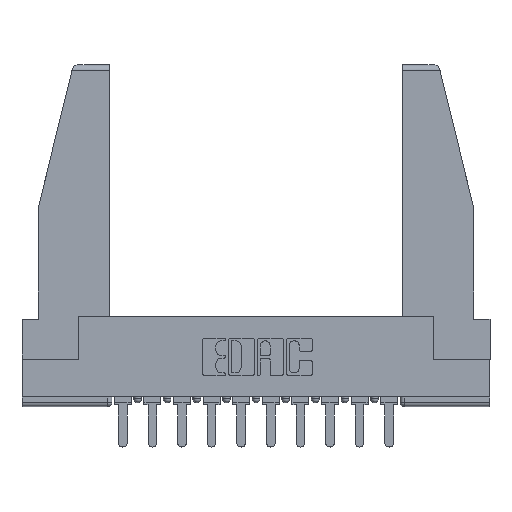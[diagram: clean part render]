
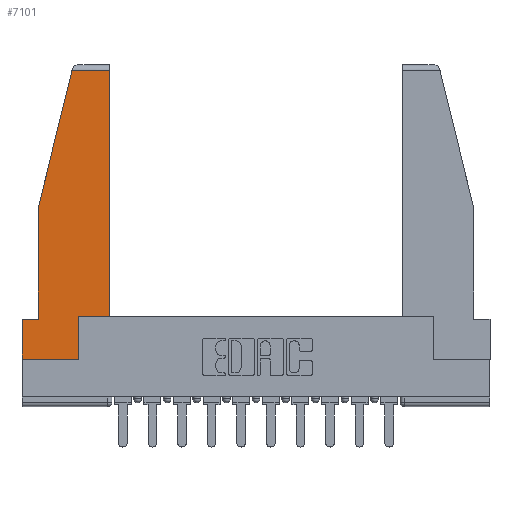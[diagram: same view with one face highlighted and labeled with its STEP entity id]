
A CAD part, top view. The second image highlights one B-rep face of the part: STEP entity #7101.
In plain terms, the highlighted planar face has unit normal (0, 0, 1).
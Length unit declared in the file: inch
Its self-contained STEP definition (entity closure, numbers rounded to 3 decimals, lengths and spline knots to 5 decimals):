
#32 = VERTEX_POINT ( 'NONE', #2172 ) ;
#370 = ORIENTED_EDGE ( 'NONE', *, *, #6871, .T. ) ;
#487 = VERTEX_POINT ( 'NONE', #7999 ) ;
#496 = DIRECTION ( 'NONE',  ( 1., 0., 0. ) ) ;
#651 = CARTESIAN_POINT ( 'NONE',  ( 0.086, 0.21, 0. ) ) ;
#810 = DIRECTION ( 'NONE',  ( 0., -1., 0. ) ) ;
#1042 = ORIENTED_EDGE ( 'NONE', *, *, #3925, .T. ) ;
#1211 = VECTOR ( 'NONE', #810, 39.37008 ) ;
#1615 = LINE ( 'NONE', #4013, #7022 ) ;
#1825 = PLANE ( 'NONE',  #9906 ) ;
#1854 = EDGE_CURVE ( 'NONE', #7035, #11301, #7400, .T. ) ;
#1891 = ORIENTED_EDGE ( 'NONE', *, *, #14746, .T. ) ;
#1901 = DIRECTION ( 'NONE',  ( 0., 0., 1. ) ) ;
#2095 = DIRECTION ( 'NONE',  ( 0., 1., 0. ) ) ;
#2172 = CARTESIAN_POINT ( 'NONE',  ( 0.461, 1.52, 0. ) ) ;
#2199 = VERTEX_POINT ( 'NONE', #10575 ) ;
#2582 = CARTESIAN_POINT ( 'NONE',  ( 0.086, 0.8, 0. ) ) ;
#2620 = DIRECTION ( 'NONE',  ( 0., -1., 0. ) ) ;
#3453 = VERTEX_POINT ( 'NONE', #15131 ) ;
#3714 = ORIENTED_EDGE ( 'NONE', *, *, #15191, .T. ) ;
#3925 = EDGE_CURVE ( 'NONE', #487, #3453, #8111, .T. ) ;
#4013 = CARTESIAN_POINT ( 'NONE',  ( 0.297, 0.223, 0. ) ) ;
#4289 = CARTESIAN_POINT ( 'NONE',  ( 0., 0., 0. ) ) ;
#4654 = VECTOR ( 'NONE', #12395, 39.37008 ) ;
#5049 = EDGE_LOOP ( 'NONE', ( #14803, #5471, #14866, #370, #12545, #3714, #12225, #1042, #1891 ) ) ;
#5052 = DIRECTION ( 'NONE',  ( 0., 1., 0. ) ) ;
#5264 = DIRECTION ( 'NONE',  ( 1., 0., 0. ) ) ;
#5281 = LINE ( 'NONE', #10124, #7884 ) ;
#5455 = DIRECTION ( 'NONE',  ( 1., 0., 0. ) ) ;
#5471 = ORIENTED_EDGE ( 'NONE', *, *, #14448, .T. ) ;
#5668 = CARTESIAN_POINT ( 'NONE',  ( 0.297, 0., 0. ) ) ;
#5722 = LINE ( 'NONE', #6760, #1211 ) ;
#5786 = EDGE_CURVE ( 'NONE', #10288, #487, #11662, .T. ) ;
#5787 = VERTEX_POINT ( 'NONE', #15323 ) ;
#6048 = CARTESIAN_POINT ( 'NONE',  ( 0.086, 0.8, 0. ) ) ;
#6076 = VERTEX_POINT ( 'NONE', #2582 ) ;
#6138 = CARTESIAN_POINT ( 'NONE',  ( 0., 0., 0. ) ) ;
#6269 = VECTOR ( 'NONE', #2095, 39.37008 ) ;
#6735 = LINE ( 'NONE', #14213, #13348 ) ;
#6760 = CARTESIAN_POINT ( 'NONE',  ( 0., 0.21, 0. ) ) ;
#6812 = DIRECTION ( 'NONE',  ( -1., 0., 0. ) ) ;
#6871 = EDGE_CURVE ( 'NONE', #6076, #7035, #11137, .T. ) ;
#6880 = CARTESIAN_POINT ( 'NONE',  ( 0., 0., 0. ) ) ;
#7022 = VECTOR ( 'NONE', #5264, 39.37008 ) ;
#7035 = VERTEX_POINT ( 'NONE', #651 ) ;
#7101 = ADVANCED_FACE ( 'NONE', ( #12695 ), #1825, .T. ) ;
#7369 = EDGE_CURVE ( 'NONE', #5787, #6076, #5281, .T. ) ;
#7400 = LINE ( 'NONE', #7563, #4654 ) ;
#7563 = CARTESIAN_POINT ( 'NONE',  ( 0., 0.21, 0. ) ) ;
#7884 = VECTOR ( 'NONE', #14996, 39.37008 ) ;
#7999 = CARTESIAN_POINT ( 'NONE',  ( 0.297, 0., 0. ) ) ;
#8111 = LINE ( 'NONE', #5668, #6269 ) ;
#9612 = VECTOR ( 'NONE', #5455, 39.37008 ) ;
#9725 = VECTOR ( 'NONE', #5052, 39.37008 ) ;
#9906 = AXIS2_PLACEMENT_3D ( 'NONE', #4289, #1901, #496 ) ;
#10124 = CARTESIAN_POINT ( 'NONE',  ( 0.271, 1.55, 0. ) ) ;
#10288 = VERTEX_POINT ( 'NONE', #6138 ) ;
#10575 = CARTESIAN_POINT ( 'NONE',  ( 0.461, 0.223, 0. ) ) ;
#11137 = LINE ( 'NONE', #6048, #13978 ) ;
#11301 = VERTEX_POINT ( 'NONE', #12149 ) ;
#11662 = LINE ( 'NONE', #6880, #9612 ) ;
#11790 = EDGE_CURVE ( 'NONE', #2199, #32, #12431, .T. ) ;
#12149 = CARTESIAN_POINT ( 'NONE',  ( 0., 0.21, 0. ) ) ;
#12225 = ORIENTED_EDGE ( 'NONE', *, *, #5786, .T. ) ;
#12395 = DIRECTION ( 'NONE',  ( -1., 0., 0. ) ) ;
#12431 = LINE ( 'NONE', #13465, #9725 ) ;
#12545 = ORIENTED_EDGE ( 'NONE', *, *, #1854, .T. ) ;
#12695 = FACE_OUTER_BOUND ( 'NONE', #5049, .T. ) ;
#13348 = VECTOR ( 'NONE', #6812, 39.37008 ) ;
#13465 = CARTESIAN_POINT ( 'NONE',  ( 0.461, 0.223, 0. ) ) ;
#13978 = VECTOR ( 'NONE', #2620, 39.37008 ) ;
#14213 = CARTESIAN_POINT ( 'NONE',  ( 0., 1.52, 0. ) ) ;
#14448 = EDGE_CURVE ( 'NONE', #32, #5787, #6735, .T. ) ;
#14746 = EDGE_CURVE ( 'NONE', #3453, #2199, #1615, .T. ) ;
#14803 = ORIENTED_EDGE ( 'NONE', *, *, #11790, .T. ) ;
#14866 = ORIENTED_EDGE ( 'NONE', *, *, #7369, .T. ) ;
#14996 = DIRECTION ( 'NONE',  ( -0.239, -0.971, 0. ) ) ;
#15131 = CARTESIAN_POINT ( 'NONE',  ( 0.297, 0.223, 0. ) ) ;
#15191 = EDGE_CURVE ( 'NONE', #11301, #10288, #5722, .T. ) ;
#15323 = CARTESIAN_POINT ( 'NONE',  ( 0.2636, 1.52, 0. ) ) ;
